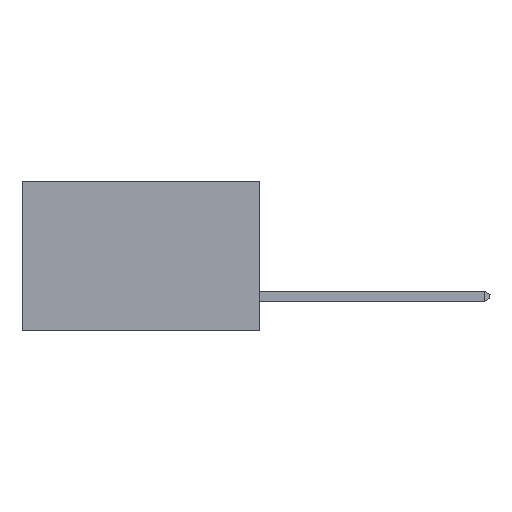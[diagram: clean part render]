
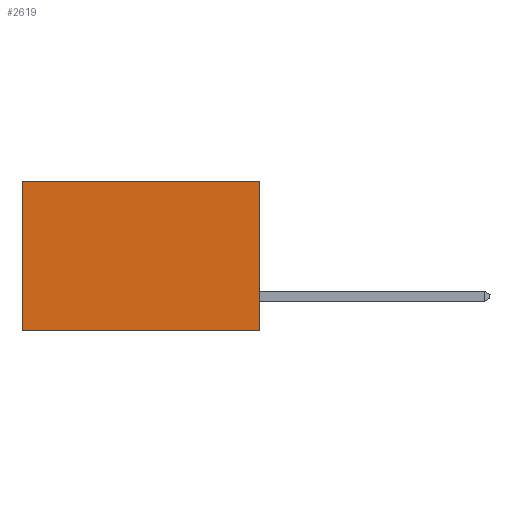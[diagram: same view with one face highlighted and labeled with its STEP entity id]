
A CAD part, left-side view. The second image highlights one B-rep face of the part: STEP entity #2619.
In plain terms, the highlighted planar face has unit normal (-1, 0, 0).
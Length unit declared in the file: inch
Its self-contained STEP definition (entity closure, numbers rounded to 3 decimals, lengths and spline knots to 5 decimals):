
#545 = VERTEX_POINT ( 'NONE', #6092 ) ;
#855 = EDGE_LOOP ( 'NONE', ( #3922, #4873, #6271, #3719 ) ) ;
#1248 = VERTEX_POINT ( 'NONE', #5753 ) ;
#1318 = EDGE_CURVE ( 'NONE', #1248, #1894, #7752, .T. ) ;
#1360 = DIRECTION ( 'NONE',  ( 0., 0., -1. ) ) ;
#1382 = DIRECTION ( 'NONE',  ( 1., 0., 0. ) ) ;
#1720 = CARTESIAN_POINT ( 'NONE',  ( 0.277, 0.59, -0.37 ) ) ;
#1894 = VERTEX_POINT ( 'NONE', #7781 ) ;
#2613 = DIRECTION ( 'NONE',  ( 0., 1., 0. ) ) ;
#2619 = ADVANCED_FACE ( 'NONE', ( #7946 ), #7998, .F. ) ;
#3604 = CARTESIAN_POINT ( 'NONE',  ( 0.277, 0., -0.37 ) ) ;
#3719 = ORIENTED_EDGE ( 'NONE', *, *, #7675, .T. ) ;
#3922 = ORIENTED_EDGE ( 'NONE', *, *, #1318, .T. ) ;
#4296 = VECTOR ( 'NONE', #7649, 39.37008 ) ;
#4331 = AXIS2_PLACEMENT_3D ( 'NONE', #3604, #1382, #1360 ) ;
#4873 = ORIENTED_EDGE ( 'NONE', *, *, #4952, .F. ) ;
#4952 = EDGE_CURVE ( 'NONE', #545, #1894, #5929, .T. ) ;
#5329 = VECTOR ( 'NONE', #8575, 39.37008 ) ;
#5753 = CARTESIAN_POINT ( 'NONE',  ( 0.277, 0.59, 0. ) ) ;
#5848 = CARTESIAN_POINT ( 'NONE',  ( 0.277, 0., 0. ) ) ;
#5929 = LINE ( 'NONE', #8473, #7337 ) ;
#6092 = CARTESIAN_POINT ( 'NONE',  ( 0.277, 0., -0.37 ) ) ;
#6271 = ORIENTED_EDGE ( 'NONE', *, *, #8098, .F. ) ;
#6730 = VERTEX_POINT ( 'NONE', #5848 ) ;
#6740 = VECTOR ( 'NONE', #8213, 39.37008 ) ;
#6957 = LINE ( 'NONE', #8225, #6740 ) ;
#7183 = LINE ( 'NONE', #9197, #5329 ) ;
#7337 = VECTOR ( 'NONE', #2613, 39.37008 ) ;
#7649 = DIRECTION ( 'NONE',  ( 0., 0., -1. ) ) ;
#7675 = EDGE_CURVE ( 'NONE', #6730, #1248, #7183, .T. ) ;
#7752 = LINE ( 'NONE', #1720, #4296 ) ;
#7781 = CARTESIAN_POINT ( 'NONE',  ( 0.277, 0.59, -0.37 ) ) ;
#7946 = FACE_OUTER_BOUND ( 'NONE', #855, .T. ) ;
#7998 = PLANE ( 'NONE',  #4331 ) ;
#8098 = EDGE_CURVE ( 'NONE', #6730, #545, #6957, .T. ) ;
#8213 = DIRECTION ( 'NONE',  ( 0., 0., -1. ) ) ;
#8225 = CARTESIAN_POINT ( 'NONE',  ( 0.277, 0., -0.37 ) ) ;
#8473 = CARTESIAN_POINT ( 'NONE',  ( 0.277, 0., -0.37 ) ) ;
#8575 = DIRECTION ( 'NONE',  ( 0., 1., 0. ) ) ;
#9197 = CARTESIAN_POINT ( 'NONE',  ( 0.277, 0., 0. ) ) ;
